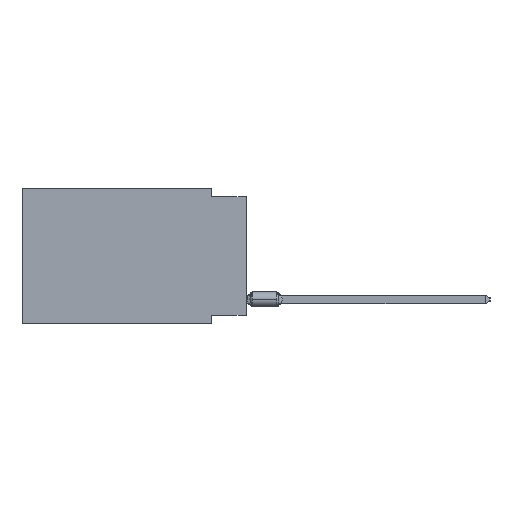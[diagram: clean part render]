
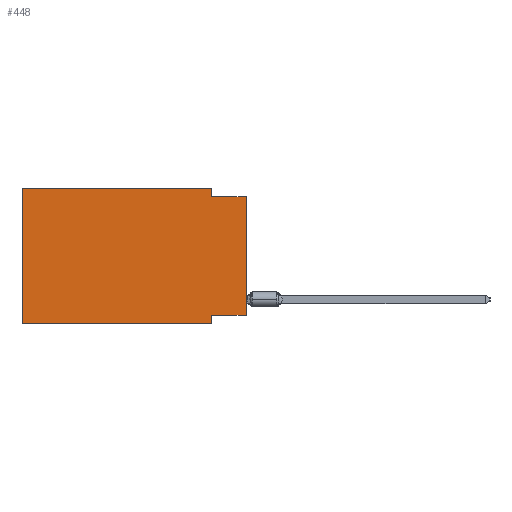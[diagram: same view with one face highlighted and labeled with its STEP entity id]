
A CAD part, left-side view. The second image highlights one B-rep face of the part: STEP entity #448.
In plain terms, the highlighted planar face has unit normal (-1, 0, 0).
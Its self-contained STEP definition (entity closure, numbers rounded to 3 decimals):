
#349 = CARTESIAN_POINT ( 'NONE',  ( 0., 2.54, -9.906 ) ) ;
#448 = ADVANCED_FACE ( 'NONE', ( #26660 ), #1691, .F. ) ;
#654 = VERTEX_POINT ( 'NONE', #15235 ) ;
#706 = EDGE_CURVE ( 'NONE', #22250, #28759, #32162, .T. ) ;
#959 = VECTOR ( 'NONE', #27717, 1000. ) ;
#1357 = EDGE_CURVE ( 'NONE', #654, #28759, #5644, .T. ) ;
#1691 = PLANE ( 'NONE',  #30816 ) ;
#1915 = VERTEX_POINT ( 'NONE', #14319 ) ;
#2049 = VECTOR ( 'NONE', #4242, 1000. ) ;
#2432 = DIRECTION ( 'NONE',  ( 0., 0., -1. ) ) ;
#2481 = VERTEX_POINT ( 'NONE', #26631 ) ;
#3378 = ORIENTED_EDGE ( 'NONE', *, *, #706, .T. ) ;
#3568 = LINE ( 'NONE', #14323, #30749 ) ;
#4242 = DIRECTION ( 'NONE',  ( 0., 1., 0. ) ) ;
#4607 = DIRECTION ( 'NONE',  ( 1., 0., 0. ) ) ;
#4709 = CARTESIAN_POINT ( 'NONE',  ( 0., 0., -9.271 ) ) ;
#5644 = LINE ( 'NONE', #11136, #10497 ) ;
#5871 = VECTOR ( 'NONE', #15964, 1000. ) ;
#5908 = CARTESIAN_POINT ( 'NONE',  ( 0., 16.383, 0. ) ) ;
#5982 = ORIENTED_EDGE ( 'NONE', *, *, #18224, .F. ) ;
#6880 = DIRECTION ( 'NONE',  ( 0., -1., 0. ) ) ;
#6935 = VERTEX_POINT ( 'NONE', #27663 ) ;
#9224 = VECTOR ( 'NONE', #6880, 1000. ) ;
#9415 = CARTESIAN_POINT ( 'NONE',  ( 0., 16.383, -9.906 ) ) ;
#9513 = ORIENTED_EDGE ( 'NONE', *, *, #31905, .F. ) ;
#9551 = CARTESIAN_POINT ( 'NONE',  ( 0., 0., -9.271 ) ) ;
#9630 = CARTESIAN_POINT ( 'NONE',  ( 0., 0., -0.635 ) ) ;
#10497 = VECTOR ( 'NONE', #2432, 1000. ) ;
#10627 = DIRECTION ( 'NONE',  ( 0., -1., 0. ) ) ;
#11136 = CARTESIAN_POINT ( 'NONE',  ( 0., 2.54, -9.906 ) ) ;
#11345 = VERTEX_POINT ( 'NONE', #4709 ) ;
#11779 = EDGE_CURVE ( 'NONE', #34356, #2481, #34950, .T. ) ;
#12119 = CARTESIAN_POINT ( 'NONE',  ( 0., 16.383, 0. ) ) ;
#14319 = CARTESIAN_POINT ( 'NONE',  ( 0., 2.54, -0.635 ) ) ;
#14323 = CARTESIAN_POINT ( 'NONE',  ( 0., 0., 0. ) ) ;
#15235 = CARTESIAN_POINT ( 'NONE',  ( 0., 2.54, -9.271 ) ) ;
#15750 = DIRECTION ( 'NONE',  ( 0., 0., -1. ) ) ;
#15964 = DIRECTION ( 'NONE',  ( 0., -1., 0. ) ) ;
#16842 = VECTOR ( 'NONE', #10627, 1000. ) ;
#16860 = DIRECTION ( 'NONE',  ( 0., 0., 1. ) ) ;
#18224 = EDGE_CURVE ( 'NONE', #11345, #654, #34687, .T. ) ;
#18466 = CARTESIAN_POINT ( 'NONE',  ( 0., 16.383, 0. ) ) ;
#18801 = CARTESIAN_POINT ( 'NONE',  ( 0., 2.54, 0. ) ) ;
#21210 = CARTESIAN_POINT ( 'NONE',  ( 0., 16.383, -9.906 ) ) ;
#22250 = VERTEX_POINT ( 'NONE', #9415 ) ;
#23316 = ORIENTED_EDGE ( 'NONE', *, *, #11779, .F. ) ;
#25205 = EDGE_CURVE ( 'NONE', #2481, #1915, #30114, .T. ) ;
#25789 = DIRECTION ( 'NONE',  ( 0., 0., 1. ) ) ;
#26533 = CARTESIAN_POINT ( 'NONE',  ( 0., 16.383, 0. ) ) ;
#26631 = CARTESIAN_POINT ( 'NONE',  ( 0., 2.54, 0. ) ) ;
#26660 = FACE_OUTER_BOUND ( 'NONE', #27100, .T. ) ;
#26714 = VECTOR ( 'NONE', #16860, 1000. ) ;
#27078 = LINE ( 'NONE', #9630, #9224 ) ;
#27100 = EDGE_LOOP ( 'NONE', ( #32406, #9513, #34819, #23316, #30211, #3378, #29716, #5982 ) ) ;
#27663 = CARTESIAN_POINT ( 'NONE',  ( 0., 0., -0.635 ) ) ;
#27717 = DIRECTION ( 'NONE',  ( 0., 0., -1. ) ) ;
#28133 = LINE ( 'NONE', #5908, #26714 ) ;
#28759 = VERTEX_POINT ( 'NONE', #349 ) ;
#29716 = ORIENTED_EDGE ( 'NONE', *, *, #1357, .F. ) ;
#30114 = LINE ( 'NONE', #18801, #959 ) ;
#30211 = ORIENTED_EDGE ( 'NONE', *, *, #33140, .F. ) ;
#30749 = VECTOR ( 'NONE', #25789, 1000. ) ;
#30816 = AXIS2_PLACEMENT_3D ( 'NONE', #18466, #4607, #15750 ) ;
#31905 = EDGE_CURVE ( 'NONE', #1915, #6935, #27078, .T. ) ;
#32162 = LINE ( 'NONE', #21210, #16842 ) ;
#32194 = EDGE_CURVE ( 'NONE', #11345, #6935, #3568, .T. ) ;
#32406 = ORIENTED_EDGE ( 'NONE', *, *, #32194, .T. ) ;
#33140 = EDGE_CURVE ( 'NONE', #22250, #34356, #28133, .T. ) ;
#34356 = VERTEX_POINT ( 'NONE', #12119 ) ;
#34687 = LINE ( 'NONE', #9551, #2049 ) ;
#34819 = ORIENTED_EDGE ( 'NONE', *, *, #25205, .F. ) ;
#34950 = LINE ( 'NONE', #26533, #5871 ) ;
